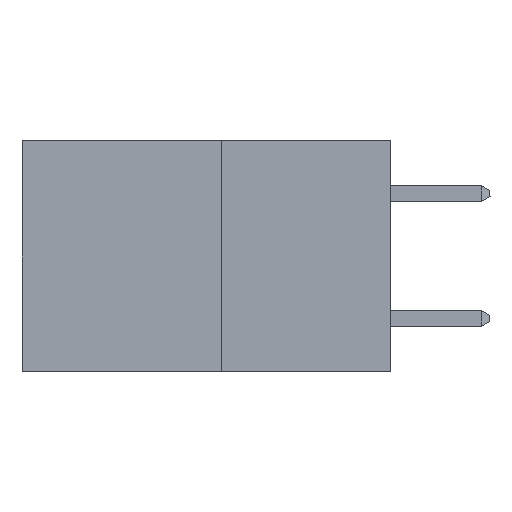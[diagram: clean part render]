
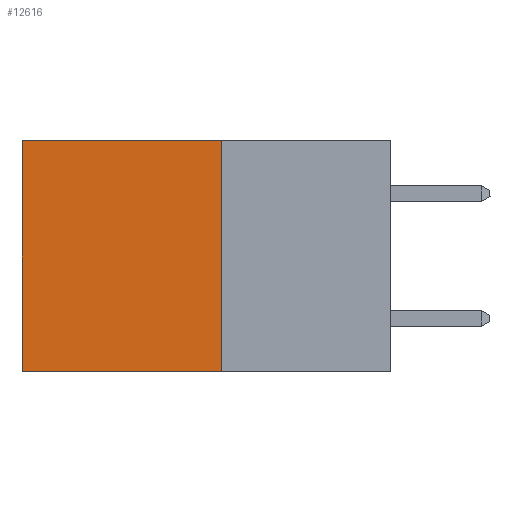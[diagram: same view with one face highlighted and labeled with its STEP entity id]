
A CAD part, left-side view. The second image highlights one B-rep face of the part: STEP entity #12616.
In plain terms, the highlighted planar face has unit normal (-1, 0, 0).
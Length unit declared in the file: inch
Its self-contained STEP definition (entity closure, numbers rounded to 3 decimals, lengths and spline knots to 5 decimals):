
#1074 = ORIENTED_EDGE ( 'NONE', *, *, #10837, .F. ) ;
#2249 = VERTEX_POINT ( 'NONE', #4260 ) ;
#3789 = EDGE_CURVE ( 'NONE', #9892, #2249, #31725, .T. ) ;
#4260 = CARTESIAN_POINT ( 'NONE',  ( 0.277, 0.27, -0.37 ) ) ;
#6089 = CARTESIAN_POINT ( 'NONE',  ( 0.277, 0.27, 0. ) ) ;
#8887 = DIRECTION ( 'NONE',  ( 0., 1., 0. ) ) ;
#9360 = CARTESIAN_POINT ( 'NONE',  ( 0.277, 0.27, -0.37 ) ) ;
#9805 = VECTOR ( 'NONE', #9833, 39.37008 ) ;
#9833 = DIRECTION ( 'NONE',  ( 0., 0., -1. ) ) ;
#9892 = VERTEX_POINT ( 'NONE', #6089 ) ;
#10146 = CARTESIAN_POINT ( 'NONE',  ( 0.277, 0.27, -0.37 ) ) ;
#10684 = LINE ( 'NONE', #22665, #24453 ) ;
#10837 = EDGE_CURVE ( 'NONE', #2249, #27462, #10684, .T. ) ;
#12154 = ORIENTED_EDGE ( 'NONE', *, *, #24006, .T. ) ;
#12616 = ADVANCED_FACE ( 'NONE', ( #18755 ), #18378, .F. ) ;
#12976 = DIRECTION ( 'NONE',  ( 0., 0., -1. ) ) ;
#13990 = CARTESIAN_POINT ( 'NONE',  ( 0.277, 0.59, 0. ) ) ;
#14981 = EDGE_LOOP ( 'NONE', ( #16267, #1074, #21504, #12154 ) ) ;
#16267 = ORIENTED_EDGE ( 'NONE', *, *, #31535, .T. ) ;
#18374 = AXIS2_PLACEMENT_3D ( 'NONE', #10146, #29358, #12976 ) ;
#18378 = PLANE ( 'NONE',  #18374 ) ;
#18755 = FACE_OUTER_BOUND ( 'NONE', #14981, .T. ) ;
#18791 = DIRECTION ( 'NONE',  ( 0., 1., 0. ) ) ;
#18860 = VERTEX_POINT ( 'NONE', #13990 ) ;
#19923 = VECTOR ( 'NONE', #18791, 39.37008 ) ;
#21504 = ORIENTED_EDGE ( 'NONE', *, *, #3789, .F. ) ;
#21511 = CARTESIAN_POINT ( 'NONE',  ( 0.277, 0.59, -0.37 ) ) ;
#21515 = VECTOR ( 'NONE', #24214, 39.37008 ) ;
#22665 = CARTESIAN_POINT ( 'NONE',  ( 0.277, 0.27, -0.37 ) ) ;
#24006 = EDGE_CURVE ( 'NONE', #9892, #18860, #27170, .T. ) ;
#24214 = DIRECTION ( 'NONE',  ( 0., 0., -1. ) ) ;
#24453 = VECTOR ( 'NONE', #8887, 39.37008 ) ;
#26905 = CARTESIAN_POINT ( 'NONE',  ( 0.277, 0.27, 0. ) ) ;
#27170 = LINE ( 'NONE', #26905, #19923 ) ;
#27462 = VERTEX_POINT ( 'NONE', #31444 ) ;
#28727 = LINE ( 'NONE', #21511, #21515 ) ;
#29358 = DIRECTION ( 'NONE',  ( 1., 0., 0. ) ) ;
#31444 = CARTESIAN_POINT ( 'NONE',  ( 0.277, 0.59, -0.37 ) ) ;
#31535 = EDGE_CURVE ( 'NONE', #18860, #27462, #28727, .T. ) ;
#31725 = LINE ( 'NONE', #9360, #9805 ) ;
